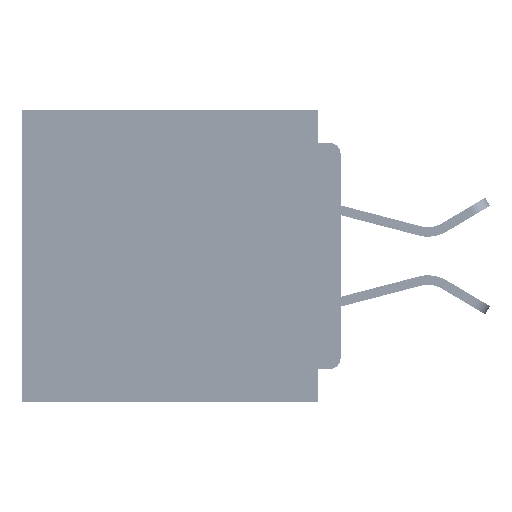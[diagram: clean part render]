
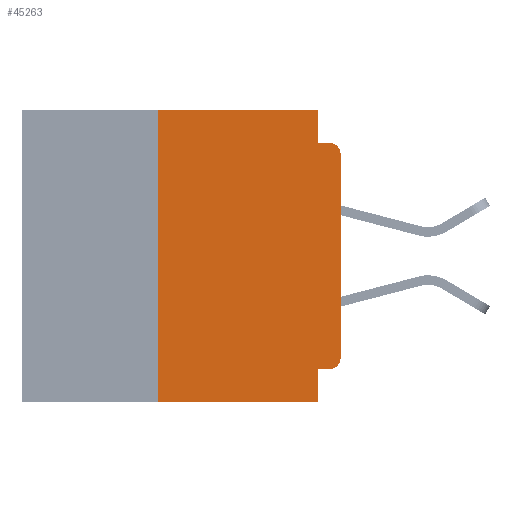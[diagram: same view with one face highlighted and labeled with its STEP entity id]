
A CAD part, left-side view. The second image highlights one B-rep face of the part: STEP entity #45263.
In plain terms, the highlighted planar face has unit normal (-1, 0, 0).
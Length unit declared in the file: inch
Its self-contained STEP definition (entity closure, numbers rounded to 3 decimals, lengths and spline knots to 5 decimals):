
#928 = DIRECTION ( 'NONE',  ( 0., 0., -1. ) ) ;
#1225 = VECTOR ( 'NONE', #20133, 39.37008 ) ;
#1324 = AXIS2_PLACEMENT_3D ( 'NONE', #59603, #29503, #64600 ) ;
#2067 = LINE ( 'NONE', #43716, #15623 ) ;
#3242 = DIRECTION ( 'NONE',  ( 0., 0., 1. ) ) ;
#7289 = VERTEX_POINT ( 'NONE', #24998 ) ;
#7369 = CARTESIAN_POINT ( 'NONE',  ( 0., 0.015, -0.06 ) ) ;
#8290 = EDGE_CURVE ( 'NONE', #13014, #60433, #56457, .T. ) ;
#8428 = VERTEX_POINT ( 'NONE', #48604 ) ;
#11462 = CARTESIAN_POINT ( 'NONE',  ( 0., 0., -0.355 ) ) ;
#11497 = CARTESIAN_POINT ( 'NONE',  ( 0., 0.031, 0. ) ) ;
#11712 = DIRECTION ( 'NONE',  ( 0., 0., -1. ) ) ;
#12454 = DIRECTION ( 'NONE',  ( 0., 0., -1. ) ) ;
#13014 = VERTEX_POINT ( 'NONE', #36205 ) ;
#13021 = ORIENTED_EDGE ( 'NONE', *, *, #37575, .T. ) ;
#13278 = ORIENTED_EDGE ( 'NONE', *, *, #61791, .F. ) ;
#13425 = CARTESIAN_POINT ( 'NONE',  ( 0., 0.25, 0. ) ) ;
#14998 = CARTESIAN_POINT ( 'NONE',  ( 0., 0.437, 0. ) ) ;
#15623 = VECTOR ( 'NONE', #3242, 39.37008 ) ;
#16537 = AXIS2_PLACEMENT_3D ( 'NONE', #26281, #31328, #928 ) ;
#16921 = EDGE_CURVE ( 'NONE', #59234, #29576, #22454, .T. ) ;
#17433 = CARTESIAN_POINT ( 'NONE',  ( 0., 0.031, -0.355 ) ) ;
#18902 = VECTOR ( 'NONE', #11712, 39.37008 ) ;
#19267 = LINE ( 'NONE', #47223, #44444 ) ;
#19543 = ORIENTED_EDGE ( 'NONE', *, *, #29199, .F. ) ;
#19976 = VECTOR ( 'NONE', #42892, 39.37008 ) ;
#20133 = DIRECTION ( 'NONE',  ( 0., -1., 0. ) ) ;
#20644 = ORIENTED_EDGE ( 'NONE', *, *, #16921, .F. ) ;
#21954 = CARTESIAN_POINT ( 'NONE',  ( 0., 0.031, -0.4 ) ) ;
#22454 = LINE ( 'NONE', #11462, #59427 ) ;
#24998 = CARTESIAN_POINT ( 'NONE',  ( 0., 0.25, -0.4 ) ) ;
#25356 = CIRCLE ( 'NONE', #1324, 0.015 ) ;
#26188 = EDGE_CURVE ( 'NONE', #7289, #28117, #2067, .T. ) ;
#26281 = CARTESIAN_POINT ( 'NONE',  ( 0., 0.437, 0. ) ) ;
#26411 = EDGE_CURVE ( 'NONE', #28117, #50799, #40048, .T. ) ;
#27113 = CARTESIAN_POINT ( 'NONE',  ( 0., 0.015, -0.355 ) ) ;
#28117 = VERTEX_POINT ( 'NONE', #13425 ) ;
#29199 = EDGE_CURVE ( 'NONE', #38094, #60433, #33341, .T. ) ;
#29503 = DIRECTION ( 'NONE',  ( -1., 0., 0. ) ) ;
#29576 = VERTEX_POINT ( 'NONE', #17433 ) ;
#31328 = DIRECTION ( 'NONE',  ( 1., 0., 0. ) ) ;
#31385 = DIRECTION ( 'NONE',  ( 0., 1., 0. ) ) ;
#32009 = CARTESIAN_POINT ( 'NONE',  ( 0., 0., 0. ) ) ;
#33341 = LINE ( 'NONE', #52790, #19976 ) ;
#34260 = CARTESIAN_POINT ( 'NONE',  ( 0., 0.031, -0.045 ) ) ;
#34728 = LINE ( 'NONE', #11497, #48119 ) ;
#36205 = CARTESIAN_POINT ( 'NONE',  ( 0., 0., -0.06 ) ) ;
#37118 = DIRECTION ( 'NONE',  ( 0., -1., 0. ) ) ;
#37430 = ORIENTED_EDGE ( 'NONE', *, *, #26188, .F. ) ;
#37575 = EDGE_CURVE ( 'NONE', #7289, #8428, #19267, .T. ) ;
#38094 = VERTEX_POINT ( 'NONE', #34260 ) ;
#38301 = VECTOR ( 'NONE', #52218, 39.37008 ) ;
#40048 = LINE ( 'NONE', #14998, #1225 ) ;
#40258 = EDGE_CURVE ( 'NONE', #29576, #8428, #45665, .T. ) ;
#41445 = LINE ( 'NONE', #32009, #38301 ) ;
#41748 = DIRECTION ( 'NONE',  ( 0., 0., -1. ) ) ;
#42692 = DIRECTION ( 'NONE',  ( -1., 0., 0. ) ) ;
#42892 = DIRECTION ( 'NONE',  ( 0., -1., 0. ) ) ;
#43009 = ORIENTED_EDGE ( 'NONE', *, *, #40258, .F. ) ;
#43716 = CARTESIAN_POINT ( 'NONE',  ( 0., 0.25, -0.4 ) ) ;
#44046 = CARTESIAN_POINT ( 'NONE',  ( 0., 0.031, 0. ) ) ;
#44444 = VECTOR ( 'NONE', #37118, 39.37008 ) ;
#45263 = ADVANCED_FACE ( 'NONE', ( #57395 ), #56399, .F. ) ;
#45546 = VERTEX_POINT ( 'NONE', #58350 ) ;
#45665 = LINE ( 'NONE', #21954, #18902 ) ;
#46721 = ORIENTED_EDGE ( 'NONE', *, *, #8290, .T. ) ;
#47223 = CARTESIAN_POINT ( 'NONE',  ( 0., 0.437, -0.4 ) ) ;
#48119 = VECTOR ( 'NONE', #41748, 39.37008 ) ;
#48604 = CARTESIAN_POINT ( 'NONE',  ( 0., 0.031, -0.4 ) ) ;
#48777 = AXIS2_PLACEMENT_3D ( 'NONE', #7369, #42692, #12454 ) ;
#49412 = EDGE_CURVE ( 'NONE', #45546, #13014, #41445, .T. ) ;
#49524 = EDGE_LOOP ( 'NONE', ( #49719, #46721, #19543, #13278, #61976, #37430, #13021, #43009, #20644, #59385 ) ) ;
#49719 = ORIENTED_EDGE ( 'NONE', *, *, #49412, .T. ) ;
#50799 = VERTEX_POINT ( 'NONE', #44046 ) ;
#52218 = DIRECTION ( 'NONE',  ( 0., 0., 1. ) ) ;
#52790 = CARTESIAN_POINT ( 'NONE',  ( 0., 0., -0.045 ) ) ;
#56399 = PLANE ( 'NONE',  #16537 ) ;
#56457 = CIRCLE ( 'NONE', #48777, 0.015 ) ;
#57395 = FACE_OUTER_BOUND ( 'NONE', #49524, .T. ) ;
#58350 = CARTESIAN_POINT ( 'NONE',  ( 0., 0., -0.34 ) ) ;
#59234 = VERTEX_POINT ( 'NONE', #27113 ) ;
#59385 = ORIENTED_EDGE ( 'NONE', *, *, #61500, .T. ) ;
#59427 = VECTOR ( 'NONE', #31385, 39.37008 ) ;
#59603 = CARTESIAN_POINT ( 'NONE',  ( 0., 0.015, -0.34 ) ) ;
#60433 = VERTEX_POINT ( 'NONE', #62968 ) ;
#61500 = EDGE_CURVE ( 'NONE', #59234, #45546, #25356, .T. ) ;
#61791 = EDGE_CURVE ( 'NONE', #50799, #38094, #34728, .T. ) ;
#61976 = ORIENTED_EDGE ( 'NONE', *, *, #26411, .F. ) ;
#62968 = CARTESIAN_POINT ( 'NONE',  ( 0., 0.015, -0.045 ) ) ;
#64600 = DIRECTION ( 'NONE',  ( 0., 0., -1. ) ) ;
